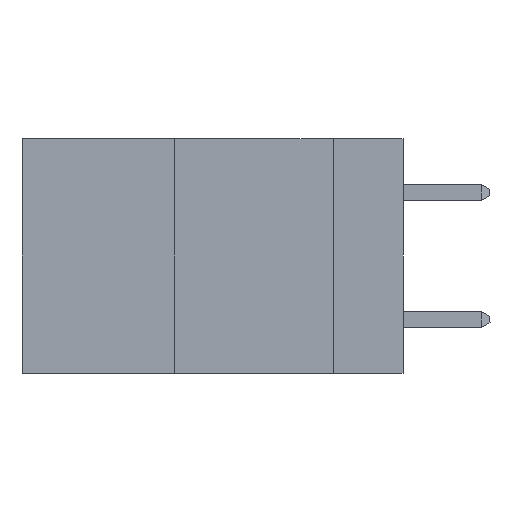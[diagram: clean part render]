
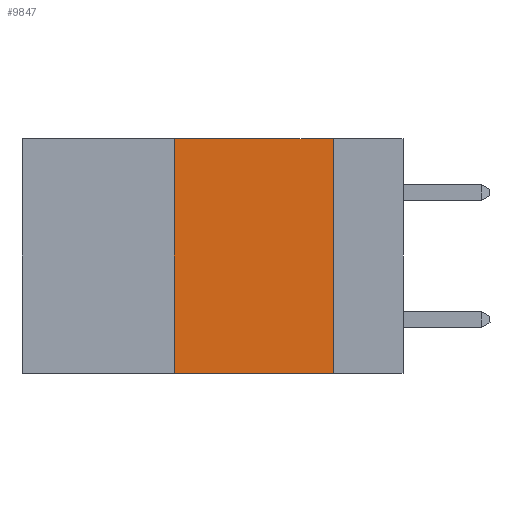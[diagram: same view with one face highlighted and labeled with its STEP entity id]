
A CAD part, left-side view. The second image highlights one B-rep face of the part: STEP entity #9847.
In plain terms, the highlighted planar face has unit normal (-1, 0, 0).
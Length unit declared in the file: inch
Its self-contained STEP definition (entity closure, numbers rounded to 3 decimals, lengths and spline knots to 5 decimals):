
#139 = ORIENTED_EDGE ( 'NONE', *, *, #14699, .T. ) ;
#434 = DIRECTION ( 'NONE',  ( 0., -1., 0. ) ) ;
#615 = PLANE ( 'NONE',  #13278 ) ;
#1428 = ORIENTED_EDGE ( 'NONE', *, *, #14348, .F. ) ;
#1901 = DIRECTION ( 'NONE',  ( 1., 0., 0. ) ) ;
#1987 = DIRECTION ( 'NONE',  ( 0., -1., 0. ) ) ;
#2394 = LINE ( 'NONE', #4866, #8692 ) ;
#3173 = EDGE_LOOP ( 'NONE', ( #3877, #1428, #9845, #139 ) ) ;
#3573 = VERTEX_POINT ( 'NONE', #13281 ) ;
#3877 = ORIENTED_EDGE ( 'NONE', *, *, #16004, .F. ) ;
#4098 = CARTESIAN_POINT ( 'NONE',  ( 0., 0.11, -0.37 ) ) ;
#4691 = CARTESIAN_POINT ( 'NONE',  ( 0., 0.11, 0. ) ) ;
#4693 = VECTOR ( 'NONE', #15725, 39.37008 ) ;
#4866 = CARTESIAN_POINT ( 'NONE',  ( 0., 0.36, 0. ) ) ;
#5700 = VERTEX_POINT ( 'NONE', #4691 ) ;
#5733 = CARTESIAN_POINT ( 'NONE',  ( 0., 0.6, 0. ) ) ;
#5756 = EDGE_CURVE ( 'NONE', #6749, #3573, #2394, .T. ) ;
#5920 = VECTOR ( 'NONE', #434, 39.37008 ) ;
#6082 = LINE ( 'NONE', #14417, #4693 ) ;
#6749 = VERTEX_POINT ( 'NONE', #14470 ) ;
#8692 = VECTOR ( 'NONE', #14868, 39.37008 ) ;
#8749 = LINE ( 'NONE', #5733, #13392 ) ;
#9845 = ORIENTED_EDGE ( 'NONE', *, *, #5756, .F. ) ;
#9847 = ADVANCED_FACE ( 'NONE', ( #15281 ), #615, .F. ) ;
#11931 = DIRECTION ( 'NONE',  ( 0., 0., -1. ) ) ;
#11987 = CARTESIAN_POINT ( 'NONE',  ( 0., 0.6, 0. ) ) ;
#13278 = AXIS2_PLACEMENT_3D ( 'NONE', #11987, #1901, #11931 ) ;
#13281 = CARTESIAN_POINT ( 'NONE',  ( 0., 0.36, 0. ) ) ;
#13392 = VECTOR ( 'NONE', #1987, 39.37008 ) ;
#14348 = EDGE_CURVE ( 'NONE', #3573, #5700, #8749, .T. ) ;
#14417 = CARTESIAN_POINT ( 'NONE',  ( 0., 0.11, 0. ) ) ;
#14470 = CARTESIAN_POINT ( 'NONE',  ( 0., 0.36, -0.37 ) ) ;
#14699 = EDGE_CURVE ( 'NONE', #6749, #15026, #15697, .T. ) ;
#14868 = DIRECTION ( 'NONE',  ( 0., 0., 1. ) ) ;
#15026 = VERTEX_POINT ( 'NONE', #4098 ) ;
#15261 = CARTESIAN_POINT ( 'NONE',  ( 0., 0.6, -0.37 ) ) ;
#15281 = FACE_OUTER_BOUND ( 'NONE', #3173, .T. ) ;
#15697 = LINE ( 'NONE', #15261, #5920 ) ;
#15725 = DIRECTION ( 'NONE',  ( 0., 0., -1. ) ) ;
#16004 = EDGE_CURVE ( 'NONE', #5700, #15026, #6082, .T. ) ;
